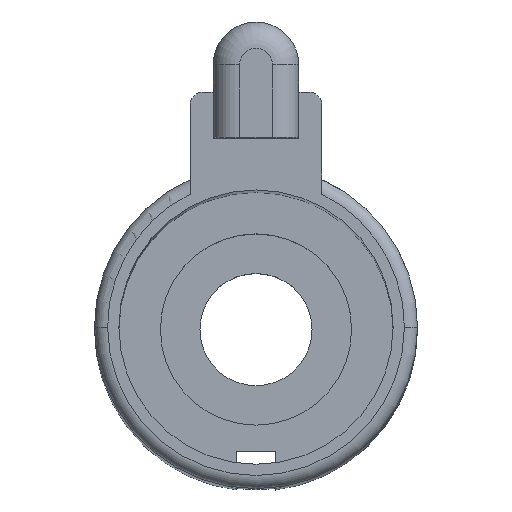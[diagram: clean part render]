
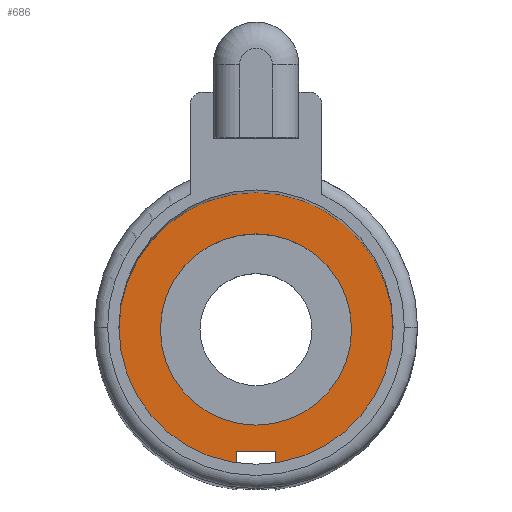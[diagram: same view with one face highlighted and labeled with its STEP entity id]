
A CAD part, top view. The second image highlights one B-rep face of the part: STEP entity #686.
In plain terms, the highlighted planar face has unit normal (0, 0, 1).
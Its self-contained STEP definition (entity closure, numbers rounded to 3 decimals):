
#3 = CARTESIAN_POINT ( 'NONE',  ( 1.5, -9.25, -104.5 ) ) ;
#26 = ORIENTED_EDGE ( 'NONE', *, *, #122, .F. ) ;
#76 = AXIS2_PLACEMENT_3D ( 'NONE', #324, #328, #1127 ) ;
#91 = EDGE_CURVE ( 'NONE', #372, #809, #625, .T. ) ;
#122 = EDGE_CURVE ( 'NONE', #1270, #233, #1403, .T. ) ;
#127 = DIRECTION ( 'NONE',  ( 1., 0., 0. ) ) ;
#144 = CARTESIAN_POINT ( 'NONE',  ( 0., -9.25, -104.5 ) ) ;
#152 = VECTOR ( 'NONE', #1058, 1000. ) ;
#195 = DIRECTION ( 'NONE',  ( 1., 0., 0. ) ) ;
#198 = EDGE_CURVE ( 'NONE', #809, #372, #592, .T. ) ;
#216 = ORIENTED_EDGE ( 'NONE', *, *, #520, .F. ) ;
#231 = FACE_BOUND ( 'NONE', #983, .T. ) ;
#233 = VERTEX_POINT ( 'NONE', #1253 ) ;
#244 = CARTESIAN_POINT ( 'NONE',  ( 10.4, 0., -104.5 ) ) ;
#247 = EDGE_LOOP ( 'NONE', ( #26, #255, #216, #371, #379, #1256 ) ) ;
#255 = ORIENTED_EDGE ( 'NONE', *, *, #478, .F. ) ;
#314 = CIRCLE ( 'NONE', #1432, 10.4 ) ;
#323 = DIRECTION ( 'NONE',  ( 0., 0., -1. ) ) ;
#324 = CARTESIAN_POINT ( 'NONE',  ( 0., 0., -104.5 ) ) ;
#328 = DIRECTION ( 'NONE',  ( 0., 0., 1. ) ) ;
#329 = VERTEX_POINT ( 'NONE', #244 ) ;
#371 = ORIENTED_EDGE ( 'NONE', *, *, #480, .F. ) ;
#372 = VERTEX_POINT ( 'NONE', #550 ) ;
#379 = ORIENTED_EDGE ( 'NONE', *, *, #702, .F. ) ;
#401 = AXIS2_PLACEMENT_3D ( 'NONE', #649, #323, #1458 ) ;
#447 = VERTEX_POINT ( 'NONE', #3 ) ;
#478 = EDGE_CURVE ( 'NONE', #447, #1270, #1074, .T. ) ;
#480 = EDGE_CURVE ( 'NONE', #329, #1369, #570, .T. ) ;
#489 = CARTESIAN_POINT ( 'NONE',  ( 1.5, 0., -104.5 ) ) ;
#520 = EDGE_CURVE ( 'NONE', #1369, #447, #863, .T. ) ;
#524 = DIRECTION ( 'NONE',  ( 0., -1., 0. ) ) ;
#550 = CARTESIAN_POINT ( 'NONE',  ( 7.25, 0., -104.5 ) ) ;
#562 = CARTESIAN_POINT ( 'NONE',  ( -7.25, 0., -104.5 ) ) ;
#570 = CIRCLE ( 'NONE', #1401, 10.4 ) ;
#592 = CIRCLE ( 'NONE', #76, 7.25 ) ;
#617 = CARTESIAN_POINT ( 'NONE',  ( 0., 0., -104.5 ) ) ;
#624 = CARTESIAN_POINT ( 'NONE',  ( -1.5, 0., -104.5 ) ) ;
#625 = CIRCLE ( 'NONE', #1293, 7.25 ) ;
#640 = EDGE_CURVE ( 'NONE', #233, #1285, #314, .T. ) ;
#649 = CARTESIAN_POINT ( 'NONE',  ( 0., 0., -104.5 ) ) ;
#686 = ADVANCED_FACE ( 'NONE', ( #1139, #231 ), #1452, .T. ) ;
#687 = CARTESIAN_POINT ( 'NONE',  ( 0., 0., -104.5 ) ) ;
#702 = EDGE_CURVE ( 'NONE', #1285, #329, #828, .T. ) ;
#740 = ORIENTED_EDGE ( 'NONE', *, *, #91, .F. ) ;
#746 = CARTESIAN_POINT ( 'NONE',  ( -1.5, -9.25, -104.5 ) ) ;
#749 = DIRECTION ( 'NONE',  ( 0., 0., 1. ) ) ;
#806 = DIRECTION ( 'NONE',  ( 0., 0., -1. ) ) ;
#809 = VERTEX_POINT ( 'NONE', #562 ) ;
#828 = CIRCLE ( 'NONE', #401, 10.4 ) ;
#863 = LINE ( 'NONE', #489, #152 ) ;
#888 = CARTESIAN_POINT ( 'NONE',  ( -10.4, 0., -104.5 ) ) ;
#918 = ORIENTED_EDGE ( 'NONE', *, *, #198, .F. ) ;
#983 = EDGE_LOOP ( 'NONE', ( #918, #740 ) ) ;
#1031 = DIRECTION ( 'NONE',  ( 0., 0., -1. ) ) ;
#1050 = CARTESIAN_POINT ( 'NONE',  ( 0., 0., -104.5 ) ) ;
#1055 = DIRECTION ( 'NONE',  ( -1., 0., 0. ) ) ;
#1058 = DIRECTION ( 'NONE',  ( 0., 1., 0. ) ) ;
#1074 = LINE ( 'NONE', #144, #1380 ) ;
#1127 = DIRECTION ( 'NONE',  ( 1., 0., 0. ) ) ;
#1139 = FACE_OUTER_BOUND ( 'NONE', #247, .T. ) ;
#1155 = DIRECTION ( 'NONE',  ( 1., 0., 0. ) ) ;
#1249 = AXIS2_PLACEMENT_3D ( 'NONE', #1327, #1338, #195 ) ;
#1253 = CARTESIAN_POINT ( 'NONE',  ( -1.5, -10.291, -104.5 ) ) ;
#1256 = ORIENTED_EDGE ( 'NONE', *, *, #640, .F. ) ;
#1270 = VERTEX_POINT ( 'NONE', #746 ) ;
#1285 = VERTEX_POINT ( 'NONE', #888 ) ;
#1293 = AXIS2_PLACEMENT_3D ( 'NONE', #617, #749, #1299 ) ;
#1299 = DIRECTION ( 'NONE',  ( 1., 0., 0. ) ) ;
#1325 = CARTESIAN_POINT ( 'NONE',  ( 1.5, -10.291, -104.5 ) ) ;
#1327 = CARTESIAN_POINT ( 'NONE',  ( 0., 0., -104.5 ) ) ;
#1328 = VECTOR ( 'NONE', #524, 1000. ) ;
#1338 = DIRECTION ( 'NONE',  ( 0., 0., 1. ) ) ;
#1369 = VERTEX_POINT ( 'NONE', #1325 ) ;
#1380 = VECTOR ( 'NONE', #1055, 1000. ) ;
#1401 = AXIS2_PLACEMENT_3D ( 'NONE', #1050, #1031, #1155 ) ;
#1403 = LINE ( 'NONE', #624, #1328 ) ;
#1432 = AXIS2_PLACEMENT_3D ( 'NONE', #687, #806, #127 ) ;
#1452 = PLANE ( 'NONE',  #1249 ) ;
#1458 = DIRECTION ( 'NONE',  ( 1., 0., 0. ) ) ;
